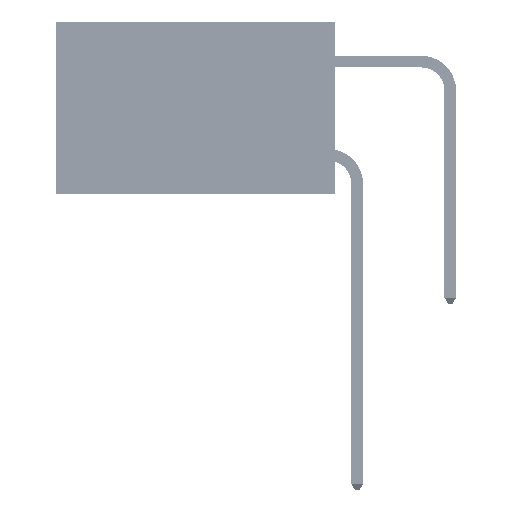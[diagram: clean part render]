
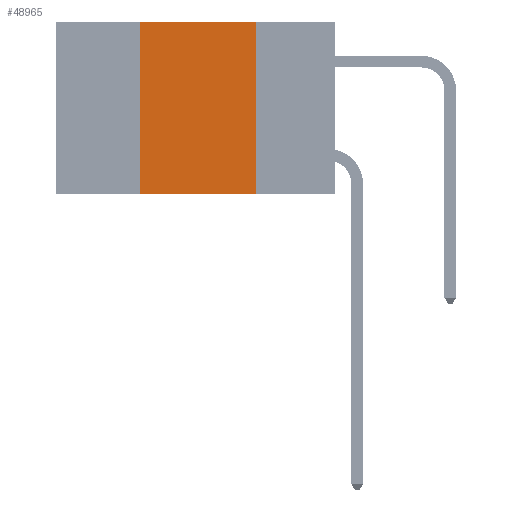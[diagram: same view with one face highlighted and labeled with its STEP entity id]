
A CAD part, left-side view. The second image highlights one B-rep face of the part: STEP entity #48965.
In plain terms, the highlighted planar face has unit normal (-1, 0, 0).
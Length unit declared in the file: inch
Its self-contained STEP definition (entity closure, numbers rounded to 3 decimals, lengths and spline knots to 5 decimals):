
#3104 = EDGE_CURVE ( 'NONE', #31077, #52538, #44692, .T. ) ;
#7183 = CARTESIAN_POINT ( 'NONE',  ( 0., 0.6, -0.37 ) ) ;
#7279 = DIRECTION ( 'NONE',  ( 0., 0., -1. ) ) ;
#10933 = LINE ( 'NONE', #7183, #32957 ) ;
#11178 = VECTOR ( 'NONE', #25688, 39.37008 ) ;
#11281 = CARTESIAN_POINT ( 'NONE',  ( 0., 0.6, 0. ) ) ;
#13392 = LINE ( 'NONE', #25168, #11178 ) ;
#13894 = LINE ( 'NONE', #46726, #38944 ) ;
#14737 = CARTESIAN_POINT ( 'NONE',  ( 0., 0.17, 0. ) ) ;
#16671 = DIRECTION ( 'NONE',  ( 0., 0., 1. ) ) ;
#19968 = VERTEX_POINT ( 'NONE', #40635 ) ;
#24348 = EDGE_CURVE ( 'NONE', #27299, #19968, #13894, .T. ) ;
#24427 = CARTESIAN_POINT ( 'NONE',  ( 0., 0.42, 0. ) ) ;
#24515 = ORIENTED_EDGE ( 'NONE', *, *, #24348, .F. ) ;
#25168 = CARTESIAN_POINT ( 'NONE',  ( 0., 0.6, 0. ) ) ;
#25178 = AXIS2_PLACEMENT_3D ( 'NONE', #11281, #43864, #7279 ) ;
#25688 = DIRECTION ( 'NONE',  ( 0., -1., 0. ) ) ;
#27299 = VERTEX_POINT ( 'NONE', #14737 ) ;
#31077 = VERTEX_POINT ( 'NONE', #37144 ) ;
#32957 = VECTOR ( 'NONE', #43514, 39.37008 ) ;
#33036 = CARTESIAN_POINT ( 'NONE',  ( 0., 0.42, 0. ) ) ;
#37144 = CARTESIAN_POINT ( 'NONE',  ( 0., 0.42, -0.37 ) ) ;
#38320 = EDGE_CURVE ( 'NONE', #31077, #19968, #10933, .T. ) ;
#38944 = VECTOR ( 'NONE', #39005, 39.37008 ) ;
#39005 = DIRECTION ( 'NONE',  ( 0., 0., -1. ) ) ;
#39341 = EDGE_LOOP ( 'NONE', ( #24515, #46678, #48357, #39462 ) ) ;
#39462 = ORIENTED_EDGE ( 'NONE', *, *, #38320, .T. ) ;
#39609 = PLANE ( 'NONE',  #25178 ) ;
#40635 = CARTESIAN_POINT ( 'NONE',  ( 0., 0.17, -0.37 ) ) ;
#43514 = DIRECTION ( 'NONE',  ( 0., -1., 0. ) ) ;
#43594 = FACE_OUTER_BOUND ( 'NONE', #39341, .T. ) ;
#43864 = DIRECTION ( 'NONE',  ( 1., 0., 0. ) ) ;
#44450 = EDGE_CURVE ( 'NONE', #52538, #27299, #13392, .T. ) ;
#44692 = LINE ( 'NONE', #24427, #45638 ) ;
#45638 = VECTOR ( 'NONE', #16671, 39.37008 ) ;
#46678 = ORIENTED_EDGE ( 'NONE', *, *, #44450, .F. ) ;
#46726 = CARTESIAN_POINT ( 'NONE',  ( 0., 0.17, 0. ) ) ;
#48357 = ORIENTED_EDGE ( 'NONE', *, *, #3104, .F. ) ;
#48965 = ADVANCED_FACE ( 'NONE', ( #43594 ), #39609, .F. ) ;
#52538 = VERTEX_POINT ( 'NONE', #33036 ) ;
